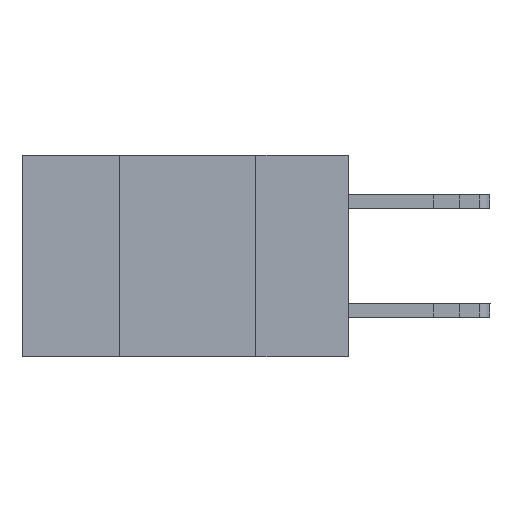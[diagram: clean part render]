
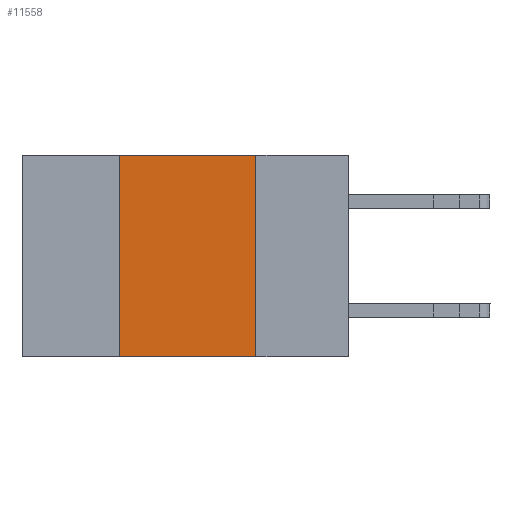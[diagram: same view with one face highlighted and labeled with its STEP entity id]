
A CAD part, left-side view. The second image highlights one B-rep face of the part: STEP entity #11558.
In plain terms, the highlighted planar face has unit normal (-1, 0, 0).
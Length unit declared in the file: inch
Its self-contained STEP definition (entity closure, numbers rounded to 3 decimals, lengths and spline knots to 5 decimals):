
#10 = VERTEX_POINT ( 'NONE', #9122 ) ;
#11 = EDGE_LOOP ( 'NONE', ( #16175, #8946, #18938, #11232 ) ) ;
#78 = DIRECTION ( 'NONE',  ( 0., 0., 1. ) ) ;
#109 = CARTESIAN_POINT ( 'NONE',  ( 0., 0.42, -0.37 ) ) ;
#604 = VECTOR ( 'NONE', #15779, 39.37008 ) ;
#988 = PLANE ( 'NONE',  #9878 ) ;
#1307 = VERTEX_POINT ( 'NONE', #7887 ) ;
#1530 = EDGE_CURVE ( 'NONE', #1307, #13529, #18859, .T. ) ;
#1763 = CARTESIAN_POINT ( 'NONE',  ( 0., 0.6, -0.37 ) ) ;
#2567 = VECTOR ( 'NONE', #6909, 39.37008 ) ;
#2722 = CARTESIAN_POINT ( 'NONE',  ( 0., 0.6, 0. ) ) ;
#2995 = CARTESIAN_POINT ( 'NONE',  ( 0., 0.42, -0.37 ) ) ;
#4329 = LINE ( 'NONE', #109, #13316 ) ;
#4442 = DIRECTION ( 'NONE',  ( 1., 0., 0. ) ) ;
#5483 = EDGE_CURVE ( 'NONE', #13529, #10, #18943, .T. ) ;
#6909 = DIRECTION ( 'NONE',  ( 0., -1., 0. ) ) ;
#6955 = EDGE_CURVE ( 'NONE', #10270, #1307, #4329, .T. ) ;
#7887 = CARTESIAN_POINT ( 'NONE',  ( 0., 0.42, 0. ) ) ;
#8665 = LINE ( 'NONE', #1763, #2567 ) ;
#8946 = ORIENTED_EDGE ( 'NONE', *, *, #1530, .F. ) ;
#9122 = CARTESIAN_POINT ( 'NONE',  ( 0., 0.17, -0.37 ) ) ;
#9878 = AXIS2_PLACEMENT_3D ( 'NONE', #2722, #4442, #16154 ) ;
#10083 = VECTOR ( 'NONE', #21247, 39.37008 ) ;
#10270 = VERTEX_POINT ( 'NONE', #2995 ) ;
#11174 = EDGE_CURVE ( 'NONE', #10270, #10, #8665, .T. ) ;
#11232 = ORIENTED_EDGE ( 'NONE', *, *, #11174, .T. ) ;
#11558 = ADVANCED_FACE ( 'NONE', ( #13133 ), #988, .F. ) ;
#13133 = FACE_OUTER_BOUND ( 'NONE', #11, .T. ) ;
#13316 = VECTOR ( 'NONE', #78, 39.37008 ) ;
#13529 = VERTEX_POINT ( 'NONE', #15609 ) ;
#15609 = CARTESIAN_POINT ( 'NONE',  ( 0., 0.17, 0. ) ) ;
#15779 = DIRECTION ( 'NONE',  ( 0., 0., -1. ) ) ;
#15879 = CARTESIAN_POINT ( 'NONE',  ( 0., 0.17, -0.37 ) ) ;
#16154 = DIRECTION ( 'NONE',  ( 0., 0., -1. ) ) ;
#16175 = ORIENTED_EDGE ( 'NONE', *, *, #5483, .F. ) ;
#18859 = LINE ( 'NONE', #21429, #10083 ) ;
#18938 = ORIENTED_EDGE ( 'NONE', *, *, #6955, .F. ) ;
#18943 = LINE ( 'NONE', #15879, #604 ) ;
#21247 = DIRECTION ( 'NONE',  ( 0., -1., 0. ) ) ;
#21429 = CARTESIAN_POINT ( 'NONE',  ( 0., 0.6, 0. ) ) ;
